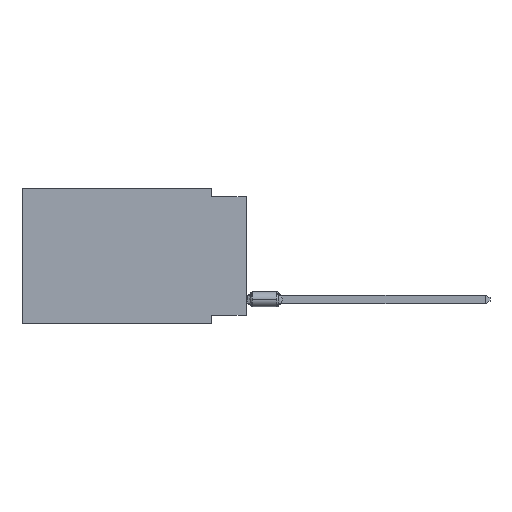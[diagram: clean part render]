
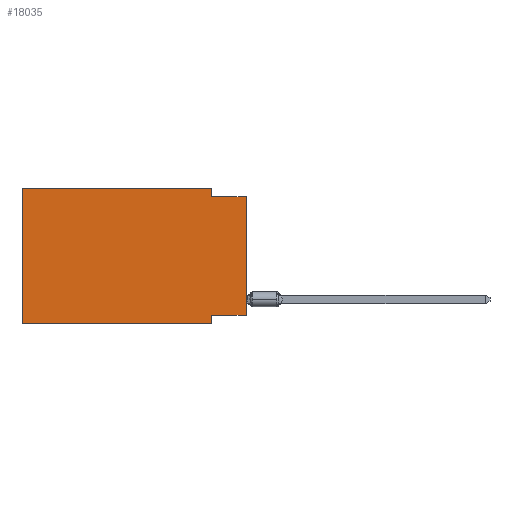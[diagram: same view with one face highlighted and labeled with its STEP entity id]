
A CAD part, left-side view. The second image highlights one B-rep face of the part: STEP entity #18035.
In plain terms, the highlighted planar face has unit normal (-1, 0, 0).
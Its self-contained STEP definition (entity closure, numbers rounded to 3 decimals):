
#172 = DIRECTION ( 'NONE',  ( 0., 1., 0. ) ) ;
#333 = CARTESIAN_POINT ( 'NONE',  ( 0., 0., -9.271 ) ) ;
#870 = ORIENTED_EDGE ( 'NONE', *, *, #8435, .T. ) ;
#891 = CARTESIAN_POINT ( 'NONE',  ( 0., 0., 0. ) ) ;
#1255 = CARTESIAN_POINT ( 'NONE',  ( 0., 16.383, 0. ) ) ;
#1340 = DIRECTION ( 'NONE',  ( 0., 0., 1. ) ) ;
#1350 = EDGE_CURVE ( 'NONE', #13397, #14420, #7914, .T. ) ;
#1606 = EDGE_CURVE ( 'NONE', #3934, #14444, #9582, .T. ) ;
#1782 = LINE ( 'NONE', #16114, #4168 ) ;
#2162 = CARTESIAN_POINT ( 'NONE',  ( 0., 16.383, -9.906 ) ) ;
#2938 = CARTESIAN_POINT ( 'NONE',  ( 0., 2.54, -9.271 ) ) ;
#3167 = VERTEX_POINT ( 'NONE', #12748 ) ;
#3934 = VERTEX_POINT ( 'NONE', #2162 ) ;
#3967 = VECTOR ( 'NONE', #9891, 1000. ) ;
#4136 = VECTOR ( 'NONE', #16038, 1000. ) ;
#4152 = LINE ( 'NONE', #9799, #3967 ) ;
#4168 = VECTOR ( 'NONE', #6118, 1000. ) ;
#4676 = DIRECTION ( 'NONE',  ( 1., 0., 0. ) ) ;
#4740 = ORIENTED_EDGE ( 'NONE', *, *, #11639, .F. ) ;
#5518 = ORIENTED_EDGE ( 'NONE', *, *, #1606, .F. ) ;
#5521 = CARTESIAN_POINT ( 'NONE',  ( 0., 0., -0.635 ) ) ;
#5700 = CARTESIAN_POINT ( 'NONE',  ( 0., 16.383, 0. ) ) ;
#6118 = DIRECTION ( 'NONE',  ( 0., -1., 0. ) ) ;
#6261 = VERTEX_POINT ( 'NONE', #12782 ) ;
#6419 = VECTOR ( 'NONE', #18156, 1000. ) ;
#6870 = ORIENTED_EDGE ( 'NONE', *, *, #1350, .T. ) ;
#7205 = ORIENTED_EDGE ( 'NONE', *, *, #15620, .F. ) ;
#7244 = PLANE ( 'NONE',  #13919 ) ;
#7694 = VECTOR ( 'NONE', #1340, 1000. ) ;
#7840 = LINE ( 'NONE', #17833, #6419 ) ;
#7914 = LINE ( 'NONE', #891, #4136 ) ;
#8435 = EDGE_CURVE ( 'NONE', #3934, #11647, #12077, .T. ) ;
#8470 = FACE_OUTER_BOUND ( 'NONE', #14385, .T. ) ;
#8595 = LINE ( 'NONE', #14219, #12511 ) ;
#9582 = LINE ( 'NONE', #1255, #7694 ) ;
#9799 = CARTESIAN_POINT ( 'NONE',  ( 0., 16.383, 0. ) ) ;
#9876 = VECTOR ( 'NONE', #11954, 1000. ) ;
#9891 = DIRECTION ( 'NONE',  ( 0., -1., 0. ) ) ;
#11048 = EDGE_CURVE ( 'NONE', #13397, #15305, #8595, .T. ) ;
#11520 = DIRECTION ( 'NONE',  ( 0., -1., 0. ) ) ;
#11540 = ORIENTED_EDGE ( 'NONE', *, *, #16886, .F. ) ;
#11639 = EDGE_CURVE ( 'NONE', #15305, #11647, #17681, .T. ) ;
#11647 = VERTEX_POINT ( 'NONE', #16106 ) ;
#11696 = DIRECTION ( 'NONE',  ( 0., 0., -1. ) ) ;
#11954 = DIRECTION ( 'NONE',  ( 0., 0., -1. ) ) ;
#12077 = LINE ( 'NONE', #12901, #15867 ) ;
#12511 = VECTOR ( 'NONE', #172, 1000. ) ;
#12748 = CARTESIAN_POINT ( 'NONE',  ( 0., 2.54, -0.635 ) ) ;
#12782 = CARTESIAN_POINT ( 'NONE',  ( 0., 2.54, 0. ) ) ;
#12882 = CARTESIAN_POINT ( 'NONE',  ( 0., 16.383, 0. ) ) ;
#12901 = CARTESIAN_POINT ( 'NONE',  ( 0., 16.383, -9.906 ) ) ;
#13397 = VERTEX_POINT ( 'NONE', #333 ) ;
#13919 = AXIS2_PLACEMENT_3D ( 'NONE', #12882, #4676, #11696 ) ;
#14044 = EDGE_CURVE ( 'NONE', #14444, #6261, #4152, .T. ) ;
#14219 = CARTESIAN_POINT ( 'NONE',  ( 0., 0., -9.271 ) ) ;
#14385 = EDGE_LOOP ( 'NONE', ( #6870, #11540, #7205, #15211, #5518, #870, #4740, #16356 ) ) ;
#14420 = VERTEX_POINT ( 'NONE', #5521 ) ;
#14444 = VERTEX_POINT ( 'NONE', #5700 ) ;
#14621 = CARTESIAN_POINT ( 'NONE',  ( 0., 2.54, -9.906 ) ) ;
#15211 = ORIENTED_EDGE ( 'NONE', *, *, #14044, .F. ) ;
#15305 = VERTEX_POINT ( 'NONE', #2938 ) ;
#15620 = EDGE_CURVE ( 'NONE', #6261, #3167, #7840, .T. ) ;
#15867 = VECTOR ( 'NONE', #11520, 1000. ) ;
#16038 = DIRECTION ( 'NONE',  ( 0., 0., 1. ) ) ;
#16106 = CARTESIAN_POINT ( 'NONE',  ( 0., 2.54, -9.906 ) ) ;
#16114 = CARTESIAN_POINT ( 'NONE',  ( 0., 0., -0.635 ) ) ;
#16356 = ORIENTED_EDGE ( 'NONE', *, *, #11048, .F. ) ;
#16886 = EDGE_CURVE ( 'NONE', #3167, #14420, #1782, .T. ) ;
#17681 = LINE ( 'NONE', #14621, #9876 ) ;
#17833 = CARTESIAN_POINT ( 'NONE',  ( 0., 2.54, 0. ) ) ;
#18035 = ADVANCED_FACE ( 'NONE', ( #8470 ), #7244, .F. ) ;
#18156 = DIRECTION ( 'NONE',  ( 0., 0., -1. ) ) ;
